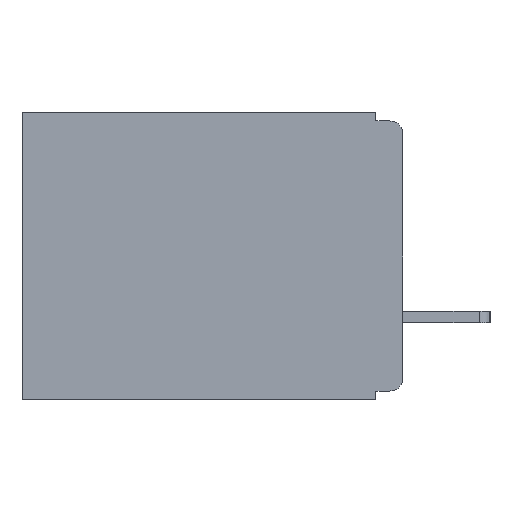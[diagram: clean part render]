
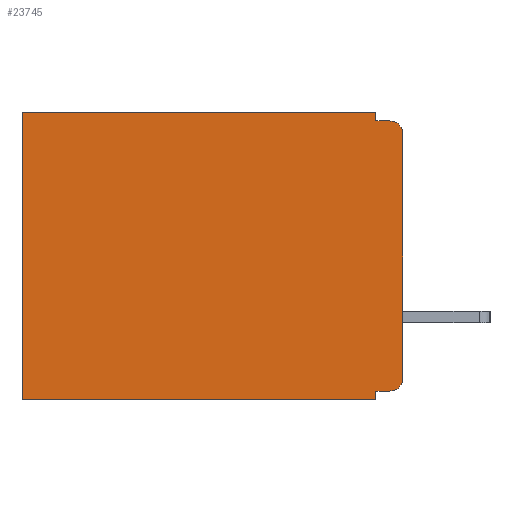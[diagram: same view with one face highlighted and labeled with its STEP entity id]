
A CAD part, left-side view. The second image highlights one B-rep face of the part: STEP entity #23745.
In plain terms, the highlighted planar face has unit normal (-1, 0, 0).
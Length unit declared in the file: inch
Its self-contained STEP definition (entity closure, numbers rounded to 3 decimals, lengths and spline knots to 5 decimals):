
#44 = CARTESIAN_POINT ( 'NONE',  ( 0.3, 0., -0.01 ) ) ;
#80 = CARTESIAN_POINT ( 'NONE',  ( 0.3, 0., -0.33 ) ) ;
#184 = EDGE_LOOP ( 'NONE', ( #20946, #7655, #4578, #17881, #22855, #10842, #23452, #23957, #10798, #18087 ) ) ;
#285 = VERTEX_POINT ( 'NONE', #20659 ) ;
#908 = CIRCLE ( 'NONE', #17381, 0.015 ) ;
#1574 = VERTEX_POINT ( 'NONE', #10040 ) ;
#1619 = CARTESIAN_POINT ( 'NONE',  ( 0.3, 0.031, -0.33 ) ) ;
#1989 = DIRECTION ( 'NONE',  ( 0., 0., -1. ) ) ;
#2073 = CARTESIAN_POINT ( 'NONE',  ( 0.3, 0.031, 0. ) ) ;
#2257 = CARTESIAN_POINT ( 'NONE',  ( 0.3, 0.437, -0.33 ) ) ;
#3244 = VECTOR ( 'NONE', #10749, 39.37008 ) ;
#3414 = AXIS2_PLACEMENT_3D ( 'NONE', #6667, #19686, #8650 ) ;
#3484 = DIRECTION ( 'NONE',  ( 0., 1., 0. ) ) ;
#3571 = CARTESIAN_POINT ( 'NONE',  ( 0.3, 0., -0.32 ) ) ;
#3647 = CARTESIAN_POINT ( 'NONE',  ( 0.3, 0.015, -0.01 ) ) ;
#3873 = VERTEX_POINT ( 'NONE', #4538 ) ;
#3987 = CARTESIAN_POINT ( 'NONE',  ( 0.3, 0.031, -0.33 ) ) ;
#4538 = CARTESIAN_POINT ( 'NONE',  ( 0.3, 0.031, -0.32 ) ) ;
#4546 = CARTESIAN_POINT ( 'NONE',  ( 0.3, 0.015, -0.305 ) ) ;
#4578 = ORIENTED_EDGE ( 'NONE', *, *, #8727, .F. ) ;
#5136 = DIRECTION ( 'NONE',  ( 0., 1., 0. ) ) ;
#5280 = DIRECTION ( 'NONE',  ( 0., 0., -1. ) ) ;
#5835 = VERTEX_POINT ( 'NONE', #8674 ) ;
#5921 = VECTOR ( 'NONE', #11608, 39.37008 ) ;
#6453 = DIRECTION ( 'NONE',  ( 0., 0., -1. ) ) ;
#6504 = VECTOR ( 'NONE', #3484, 39.37008 ) ;
#6571 = EDGE_CURVE ( 'NONE', #15130, #17227, #14639, .T. ) ;
#6659 = VECTOR ( 'NONE', #5136, 39.37008 ) ;
#6667 = CARTESIAN_POINT ( 'NONE',  ( 0.3, 0.015, -0.025 ) ) ;
#7276 = LINE ( 'NONE', #20038, #6659 ) ;
#7335 = FACE_OUTER_BOUND ( 'NONE', #184, .T. ) ;
#7655 = ORIENTED_EDGE ( 'NONE', *, *, #11336, .T. ) ;
#7692 = CIRCLE ( 'NONE', #3414, 0.015 ) ;
#7968 = VERTEX_POINT ( 'NONE', #20405 ) ;
#8272 = CARTESIAN_POINT ( 'NONE',  ( 0.3, 0.437, 0. ) ) ;
#8334 = LINE ( 'NONE', #17994, #3244 ) ;
#8650 = DIRECTION ( 'NONE',  ( 0., 0., -1. ) ) ;
#8674 = CARTESIAN_POINT ( 'NONE',  ( 0.3, 0.031, -0.01 ) ) ;
#8723 = VECTOR ( 'NONE', #17110, 39.37008 ) ;
#8727 = EDGE_CURVE ( 'NONE', #5835, #13222, #16583, .T. ) ;
#9042 = CARTESIAN_POINT ( 'NONE',  ( 0.3, 0., -0.33 ) ) ;
#9297 = EDGE_CURVE ( 'NONE', #3873, #15130, #22845, .T. ) ;
#10040 = CARTESIAN_POINT ( 'NONE',  ( 0.3, 0.031, 0. ) ) ;
#10439 = EDGE_CURVE ( 'NONE', #1574, #5835, #11036, .T. ) ;
#10749 = DIRECTION ( 'NONE',  ( 0., 0., -1. ) ) ;
#10791 = EDGE_CURVE ( 'NONE', #7968, #285, #8334, .T. ) ;
#10798 = ORIENTED_EDGE ( 'NONE', *, *, #22237, .F. ) ;
#10842 = ORIENTED_EDGE ( 'NONE', *, *, #20915, .T. ) ;
#11036 = LINE ( 'NONE', #2073, #5921 ) ;
#11041 = LINE ( 'NONE', #3571, #6504 ) ;
#11336 = EDGE_CURVE ( 'NONE', #7968, #13222, #7692, .T. ) ;
#11437 = PLANE ( 'NONE',  #19955 ) ;
#11608 = DIRECTION ( 'NONE',  ( 0., 0., -1. ) ) ;
#12301 = VECTOR ( 'NONE', #13670, 39.37008 ) ;
#12916 = EDGE_CURVE ( 'NONE', #17160, #285, #908, .T. ) ;
#13222 = VERTEX_POINT ( 'NONE', #3647 ) ;
#13275 = DIRECTION ( 'NONE',  ( 1., 0., 0. ) ) ;
#13670 = DIRECTION ( 'NONE',  ( 0., -1., 0. ) ) ;
#14639 = LINE ( 'NONE', #9042, #18953 ) ;
#15130 = VERTEX_POINT ( 'NONE', #1619 ) ;
#15722 = DIRECTION ( 'NONE',  ( 0., 1., 0. ) ) ;
#16232 = LINE ( 'NONE', #16529, #20514 ) ;
#16529 = CARTESIAN_POINT ( 'NONE',  ( 0.3, 0.437, -0.33 ) ) ;
#16583 = LINE ( 'NONE', #44, #12301 ) ;
#16935 = CARTESIAN_POINT ( 'NONE',  ( 0.3, 0.015, -0.32 ) ) ;
#17110 = DIRECTION ( 'NONE',  ( 0., 0., -1. ) ) ;
#17160 = VERTEX_POINT ( 'NONE', #16935 ) ;
#17227 = VERTEX_POINT ( 'NONE', #2257 ) ;
#17381 = AXIS2_PLACEMENT_3D ( 'NONE', #4546, #17669, #6453 ) ;
#17669 = DIRECTION ( 'NONE',  ( -1., 0., 0. ) ) ;
#17881 = ORIENTED_EDGE ( 'NONE', *, *, #10439, .F. ) ;
#17994 = CARTESIAN_POINT ( 'NONE',  ( 0.3, 0., -0.33 ) ) ;
#18087 = ORIENTED_EDGE ( 'NONE', *, *, #12916, .T. ) ;
#18372 = VERTEX_POINT ( 'NONE', #8272 ) ;
#18588 = EDGE_CURVE ( 'NONE', #1574, #18372, #7276, .T. ) ;
#18953 = VECTOR ( 'NONE', #15722, 39.37008 ) ;
#19686 = DIRECTION ( 'NONE',  ( -1., 0., 0. ) ) ;
#19955 = AXIS2_PLACEMENT_3D ( 'NONE', #80, #13275, #1989 ) ;
#20038 = CARTESIAN_POINT ( 'NONE',  ( 0.3, 0., 0. ) ) ;
#20405 = CARTESIAN_POINT ( 'NONE',  ( 0.3, 0., -0.025 ) ) ;
#20514 = VECTOR ( 'NONE', #5280, 39.37008 ) ;
#20659 = CARTESIAN_POINT ( 'NONE',  ( 0.3, 0., -0.305 ) ) ;
#20915 = EDGE_CURVE ( 'NONE', #18372, #17227, #16232, .T. ) ;
#20946 = ORIENTED_EDGE ( 'NONE', *, *, #10791, .F. ) ;
#22237 = EDGE_CURVE ( 'NONE', #17160, #3873, #11041, .T. ) ;
#22845 = LINE ( 'NONE', #3987, #8723 ) ;
#22855 = ORIENTED_EDGE ( 'NONE', *, *, #18588, .T. ) ;
#23452 = ORIENTED_EDGE ( 'NONE', *, *, #6571, .F. ) ;
#23745 = ADVANCED_FACE ( 'NONE', ( #7335 ), #11437, .F. ) ;
#23957 = ORIENTED_EDGE ( 'NONE', *, *, #9297, .F. ) ;
